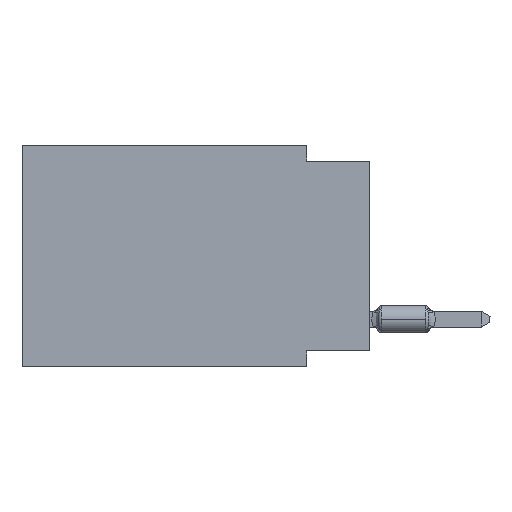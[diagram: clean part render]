
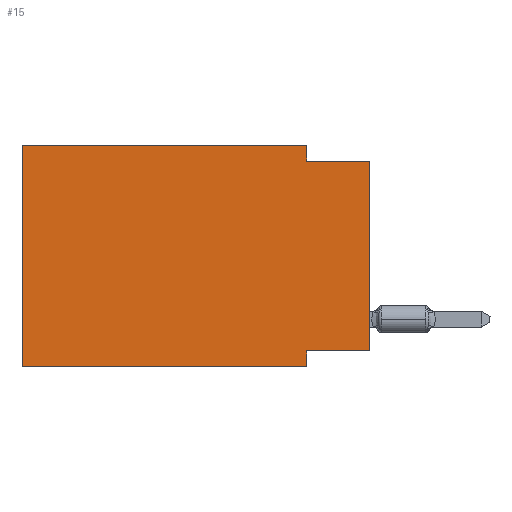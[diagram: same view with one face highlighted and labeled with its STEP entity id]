
A CAD part, left-side view. The second image highlights one B-rep face of the part: STEP entity #15.
In plain terms, the highlighted planar face has unit normal (-1, 0, 0).
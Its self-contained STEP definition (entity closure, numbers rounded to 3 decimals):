
#15 = ADVANCED_FACE ( 'NONE', ( #12584 ), #57779, .F. ) ;
#1106 = CARTESIAN_POINT ( 'NONE',  ( 0., 0., -8.255 ) ) ;
#1561 = EDGE_CURVE ( 'NONE', #5559, #6841, #43343, .T. ) ;
#1635 = ORIENTED_EDGE ( 'NONE', *, *, #28731, .F. ) ;
#2895 = LINE ( 'NONE', #32368, #4559 ) ;
#3937 = EDGE_CURVE ( 'NONE', #43895, #6841, #45064, .T. ) ;
#4559 = VECTOR ( 'NONE', #31997, 1000. ) ;
#5559 = VERTEX_POINT ( 'NONE', #50966 ) ;
#5609 = DIRECTION ( 'NONE',  ( 0., 0., -1. ) ) ;
#5886 = LINE ( 'NONE', #69371, #22146 ) ;
#6833 = VECTOR ( 'NONE', #5609, 1000. ) ;
#6841 = VERTEX_POINT ( 'NONE', #34767 ) ;
#7333 = ORIENTED_EDGE ( 'NONE', *, *, #57619, .F. ) ;
#7343 = DIRECTION ( 'NONE',  ( 1., 0., 0. ) ) ;
#7554 = ORIENTED_EDGE ( 'NONE', *, *, #41185, .T. ) ;
#8623 = DIRECTION ( 'NONE',  ( 0., -1., 0. ) ) ;
#10054 = ORIENTED_EDGE ( 'NONE', *, *, #3937, .T. ) ;
#10739 = LINE ( 'NONE', #17075, #28129 ) ;
#11087 = DIRECTION ( 'NONE',  ( 0., 0., 1. ) ) ;
#11213 = ORIENTED_EDGE ( 'NONE', *, *, #25058, .F. ) ;
#11775 = VECTOR ( 'NONE', #41569, 1000. ) ;
#12584 = FACE_OUTER_BOUND ( 'NONE', #67232, .T. ) ;
#12950 = CARTESIAN_POINT ( 'NONE',  ( 0., 13.97, 0. ) ) ;
#17075 = CARTESIAN_POINT ( 'NONE',  ( 0., 13.97, -8.89 ) ) ;
#19434 = ORIENTED_EDGE ( 'NONE', *, *, #1561, .F. ) ;
#20175 = CARTESIAN_POINT ( 'NONE',  ( 0., 0., -0.635 ) ) ;
#21642 = LINE ( 'NONE', #44430, #36008 ) ;
#22146 = VECTOR ( 'NONE', #45478, 1000. ) ;
#23734 = CARTESIAN_POINT ( 'NONE',  ( 0., 2.54, 0. ) ) ;
#24745 = CARTESIAN_POINT ( 'NONE',  ( 0., 13.97, 0. ) ) ;
#25058 = EDGE_CURVE ( 'NONE', #73143, #5559, #5886, .T. ) ;
#28129 = VECTOR ( 'NONE', #40596, 1000. ) ;
#28731 = EDGE_CURVE ( 'NONE', #33189, #38045, #32522, .T. ) ;
#31997 = DIRECTION ( 'NONE',  ( 0., 1., 0. ) ) ;
#32368 = CARTESIAN_POINT ( 'NONE',  ( 0., 0., -8.255 ) ) ;
#32522 = LINE ( 'NONE', #50067, #6833 ) ;
#33189 = VERTEX_POINT ( 'NONE', #55699 ) ;
#34767 = CARTESIAN_POINT ( 'NONE',  ( 0., 0., -0.635 ) ) ;
#35608 = LINE ( 'NONE', #24745, #11775 ) ;
#36008 = VECTOR ( 'NONE', #72096, 1000. ) ;
#36979 = CARTESIAN_POINT ( 'NONE',  ( 0., 13.97, -8.89 ) ) ;
#38045 = VERTEX_POINT ( 'NONE', #42861 ) ;
#40596 = DIRECTION ( 'NONE',  ( 0., -1., 0. ) ) ;
#41185 = EDGE_CURVE ( 'NONE', #61371, #38045, #10739, .T. ) ;
#41569 = DIRECTION ( 'NONE',  ( 0., 0., 1. ) ) ;
#42861 = CARTESIAN_POINT ( 'NONE',  ( 0., 2.54, -8.89 ) ) ;
#43343 = LINE ( 'NONE', #20175, #61269 ) ;
#43895 = VERTEX_POINT ( 'NONE', #1106 ) ;
#44430 = CARTESIAN_POINT ( 'NONE',  ( 0., 13.97, 0. ) ) ;
#45064 = LINE ( 'NONE', #62244, #45604 ) ;
#45359 = ORIENTED_EDGE ( 'NONE', *, *, #49310, .F. ) ;
#45478 = DIRECTION ( 'NONE',  ( 0., 0., -1. ) ) ;
#45604 = VECTOR ( 'NONE', #11087, 1000. ) ;
#47522 = VERTEX_POINT ( 'NONE', #66939 ) ;
#49310 = EDGE_CURVE ( 'NONE', #47522, #73143, #21642, .T. ) ;
#50067 = CARTESIAN_POINT ( 'NONE',  ( 0., 2.54, -8.89 ) ) ;
#50966 = CARTESIAN_POINT ( 'NONE',  ( 0., 2.54, -0.635 ) ) ;
#53977 = AXIS2_PLACEMENT_3D ( 'NONE', #12950, #7343, #63760 ) ;
#55699 = CARTESIAN_POINT ( 'NONE',  ( 0., 2.54, -8.255 ) ) ;
#57619 = EDGE_CURVE ( 'NONE', #43895, #33189, #2895, .T. ) ;
#57779 = PLANE ( 'NONE',  #53977 ) ;
#61269 = VECTOR ( 'NONE', #8623, 1000. ) ;
#61371 = VERTEX_POINT ( 'NONE', #36979 ) ;
#61547 = ORIENTED_EDGE ( 'NONE', *, *, #65615, .F. ) ;
#62244 = CARTESIAN_POINT ( 'NONE',  ( 0., 0., 0. ) ) ;
#63760 = DIRECTION ( 'NONE',  ( 0., 0., -1. ) ) ;
#65615 = EDGE_CURVE ( 'NONE', #61371, #47522, #35608, .T. ) ;
#66939 = CARTESIAN_POINT ( 'NONE',  ( 0., 13.97, 0. ) ) ;
#67232 = EDGE_LOOP ( 'NONE', ( #10054, #19434, #11213, #45359, #61547, #7554, #1635, #7333 ) ) ;
#69371 = CARTESIAN_POINT ( 'NONE',  ( 0., 2.54, 0. ) ) ;
#72096 = DIRECTION ( 'NONE',  ( 0., -1., 0. ) ) ;
#73143 = VERTEX_POINT ( 'NONE', #23734 ) ;
